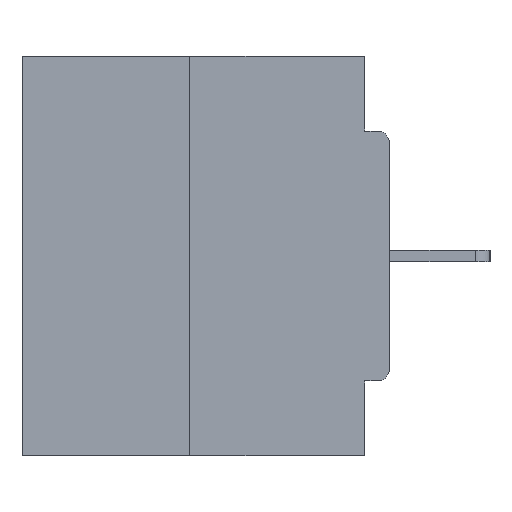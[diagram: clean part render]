
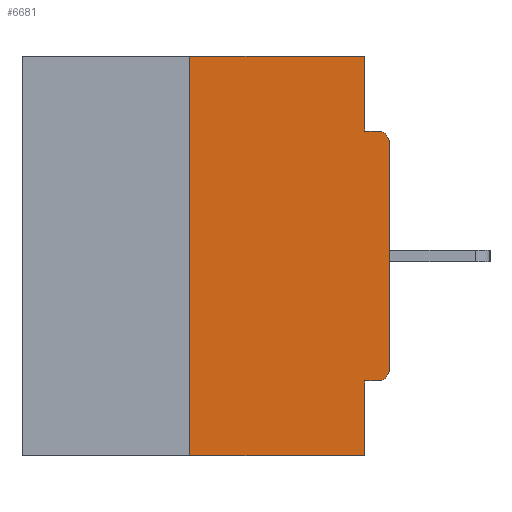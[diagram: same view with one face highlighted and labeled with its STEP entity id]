
A CAD part, left-side view. The second image highlights one B-rep face of the part: STEP entity #6681.
In plain terms, the highlighted planar face has unit normal (-1, 0, 0).
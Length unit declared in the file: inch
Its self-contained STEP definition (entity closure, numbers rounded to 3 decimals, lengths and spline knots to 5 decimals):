
#54 = AXIS2_PLACEMENT_3D ( 'NONE', #27563, #14141, #29823 ) ;
#354 = EDGE_CURVE ( 'NONE', #10560, #11973, #2893, .T. ) ;
#766 = CARTESIAN_POINT ( 'NONE',  ( 0., 0.015, -0.1085 ) ) ;
#1334 = ORIENTED_EDGE ( 'NONE', *, *, #10372, .F. ) ;
#2333 = DIRECTION ( 'NONE',  ( 0., -1., 0. ) ) ;
#2356 = CARTESIAN_POINT ( 'NONE',  ( 0., 0.031, -0.0935 ) ) ;
#2590 = VERTEX_POINT ( 'NONE', #29029 ) ;
#2634 = VECTOR ( 'NONE', #21209, 39.37008 ) ;
#2638 = CARTESIAN_POINT ( 'NONE',  ( 0., 0.031, -0.5 ) ) ;
#2893 = LINE ( 'NONE', #19458, #8470 ) ;
#3213 = DIRECTION ( 'NONE',  ( 0., 0., -1. ) ) ;
#3886 = AXIS2_PLACEMENT_3D ( 'NONE', #24462, #10892, #26708 ) ;
#4017 = EDGE_CURVE ( 'NONE', #17656, #2590, #4153, .T. ) ;
#4078 = EDGE_CURVE ( 'NONE', #11973, #28920, #26391, .T. ) ;
#4153 = LINE ( 'NONE', #4675, #21862 ) ;
#4484 = DIRECTION ( 'NONE',  ( 0., 0., 1. ) ) ;
#4675 = CARTESIAN_POINT ( 'NONE',  ( 0., 0., -0.0935 ) ) ;
#5627 = ORIENTED_EDGE ( 'NONE', *, *, #27619, .T. ) ;
#6511 = CARTESIAN_POINT ( 'NONE',  ( 0., 0.031, -0.4065 ) ) ;
#6659 = ORIENTED_EDGE ( 'NONE', *, *, #354, .F. ) ;
#6681 = ADVANCED_FACE ( 'NONE', ( #14061 ), #16306, .F. ) ;
#6722 = DIRECTION ( 'NONE',  ( 0., 0., 1. ) ) ;
#7350 = DIRECTION ( 'NONE',  ( 0., -1., 0. ) ) ;
#8270 = CARTESIAN_POINT ( 'NONE',  ( 0., 0.46, -0.5 ) ) ;
#8470 = VECTOR ( 'NONE', #4484, 39.37008 ) ;
#8969 = LINE ( 'NONE', #2638, #2634 ) ;
#9435 = VECTOR ( 'NONE', #29192, 39.37008 ) ;
#9458 = LINE ( 'NONE', #8270, #26828 ) ;
#9659 = VERTEX_POINT ( 'NONE', #6511 ) ;
#10372 = EDGE_CURVE ( 'NONE', #22831, #9659, #27184, .T. ) ;
#10381 = CARTESIAN_POINT ( 'NONE',  ( 0., 0.031, -0.5 ) ) ;
#10560 = VERTEX_POINT ( 'NONE', #23694 ) ;
#10743 = DIRECTION ( 'NONE',  ( 0., -1., 0. ) ) ;
#10892 = DIRECTION ( 'NONE',  ( -1., 0., 0. ) ) ;
#11150 = VECTOR ( 'NONE', #6722, 39.37008 ) ;
#11152 = EDGE_LOOP ( 'NONE', ( #12855, #6659, #14847, #15493, #1334, #5627, #14495, #13602, #27233, #21020 ) ) ;
#11370 = VERTEX_POINT ( 'NONE', #10381 ) ;
#11973 = VERTEX_POINT ( 'NONE', #28657 ) ;
#12855 = ORIENTED_EDGE ( 'NONE', *, *, #4078, .F. ) ;
#13497 = CARTESIAN_POINT ( 'NONE',  ( 0., 0.031, 0. ) ) ;
#13602 = ORIENTED_EDGE ( 'NONE', *, *, #21642, .T. ) ;
#13774 = VECTOR ( 'NONE', #7350, 39.37008 ) ;
#13994 = CARTESIAN_POINT ( 'NONE',  ( 0., 0., -0.4065 ) ) ;
#14061 = FACE_OUTER_BOUND ( 'NONE', #11152, .T. ) ;
#14141 = DIRECTION ( 'NONE',  ( 1., 0., 0. ) ) ;
#14495 = ORIENTED_EDGE ( 'NONE', *, *, #18079, .T. ) ;
#14847 = ORIENTED_EDGE ( 'NONE', *, *, #24241, .T. ) ;
#14860 = AXIS2_PLACEMENT_3D ( 'NONE', #766, #17217, #3213 ) ;
#15296 = CARTESIAN_POINT ( 'NONE',  ( 0., 0.031, 0. ) ) ;
#15493 = ORIENTED_EDGE ( 'NONE', *, *, #22739, .F. ) ;
#16306 = PLANE ( 'NONE',  #54 ) ;
#16609 = CARTESIAN_POINT ( 'NONE',  ( 0., 0.46, 0. ) ) ;
#17067 = CARTESIAN_POINT ( 'NONE',  ( 0., 0.015, -0.4065 ) ) ;
#17217 = DIRECTION ( 'NONE',  ( -1., 0., 0. ) ) ;
#17656 = VERTEX_POINT ( 'NONE', #2356 ) ;
#17695 = CIRCLE ( 'NONE', #14860, 0.015 ) ;
#18079 = EDGE_CURVE ( 'NONE', #18125, #21955, #24598, .T. ) ;
#18125 = VERTEX_POINT ( 'NONE', #29630 ) ;
#18297 = CARTESIAN_POINT ( 'NONE',  ( 0., 0., 0. ) ) ;
#19458 = CARTESIAN_POINT ( 'NONE',  ( 0., 0.25, 0. ) ) ;
#20192 = LINE ( 'NONE', #13497, #9435 ) ;
#21020 = ORIENTED_EDGE ( 'NONE', *, *, #21261, .F. ) ;
#21052 = CARTESIAN_POINT ( 'NONE',  ( 0., 0., -0.1085 ) ) ;
#21209 = DIRECTION ( 'NONE',  ( 0., 0., -1. ) ) ;
#21261 = EDGE_CURVE ( 'NONE', #28920, #17656, #20192, .T. ) ;
#21277 = VECTOR ( 'NONE', #22999, 39.37008 ) ;
#21642 = EDGE_CURVE ( 'NONE', #21955, #2590, #17695, .T. ) ;
#21862 = VECTOR ( 'NONE', #2333, 39.37008 ) ;
#21955 = VERTEX_POINT ( 'NONE', #21052 ) ;
#22739 = EDGE_CURVE ( 'NONE', #9659, #11370, #8969, .T. ) ;
#22831 = VERTEX_POINT ( 'NONE', #17067 ) ;
#22999 = DIRECTION ( 'NONE',  ( 0., 1., 0. ) ) ;
#23694 = CARTESIAN_POINT ( 'NONE',  ( 0., 0.25, -0.5 ) ) ;
#24241 = EDGE_CURVE ( 'NONE', #10560, #11370, #9458, .T. ) ;
#24462 = CARTESIAN_POINT ( 'NONE',  ( 0., 0.015, -0.3915 ) ) ;
#24598 = LINE ( 'NONE', #18297, #11150 ) ;
#26391 = LINE ( 'NONE', #16609, #13774 ) ;
#26708 = DIRECTION ( 'NONE',  ( 0., 0., -1. ) ) ;
#26828 = VECTOR ( 'NONE', #10743, 39.37008 ) ;
#27184 = LINE ( 'NONE', #13994, #21277 ) ;
#27233 = ORIENTED_EDGE ( 'NONE', *, *, #4017, .F. ) ;
#27563 = CARTESIAN_POINT ( 'NONE',  ( 0., 0.46, 0. ) ) ;
#27619 = EDGE_CURVE ( 'NONE', #22831, #18125, #28440, .T. ) ;
#28440 = CIRCLE ( 'NONE', #3886, 0.015 ) ;
#28657 = CARTESIAN_POINT ( 'NONE',  ( 0., 0.25, 0. ) ) ;
#28920 = VERTEX_POINT ( 'NONE', #15296 ) ;
#29029 = CARTESIAN_POINT ( 'NONE',  ( 0., 0.015, -0.0935 ) ) ;
#29192 = DIRECTION ( 'NONE',  ( 0., 0., -1. ) ) ;
#29630 = CARTESIAN_POINT ( 'NONE',  ( 0., 0., -0.3915 ) ) ;
#29823 = DIRECTION ( 'NONE',  ( 0., 0., -1. ) ) ;
